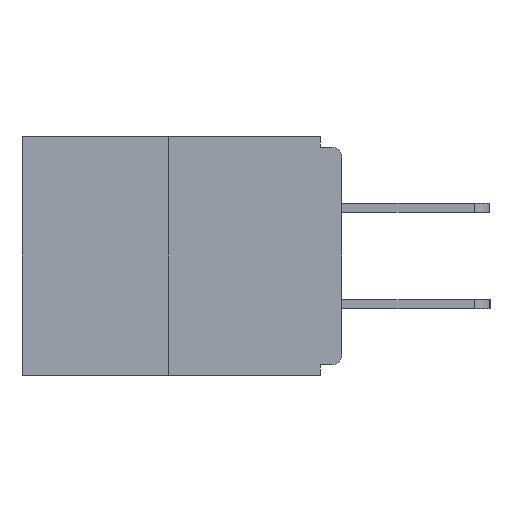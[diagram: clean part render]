
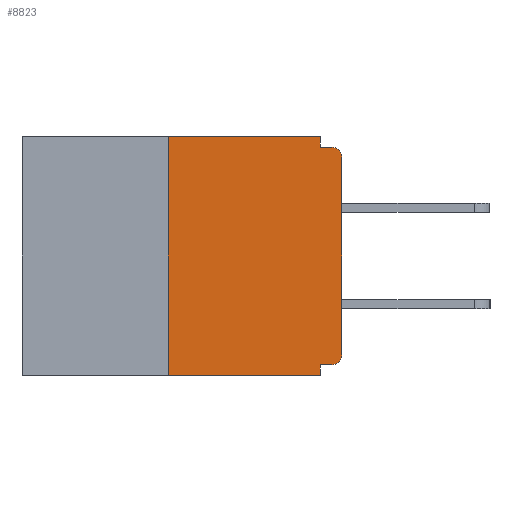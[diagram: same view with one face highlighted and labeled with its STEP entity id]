
A CAD part, left-side view. The second image highlights one B-rep face of the part: STEP entity #8823.
In plain terms, the highlighted planar face has unit normal (-1, 0, 0).
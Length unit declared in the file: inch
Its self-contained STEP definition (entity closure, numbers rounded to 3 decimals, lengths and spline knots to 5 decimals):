
#463 = ORIENTED_EDGE ( 'NONE', *, *, #13800, .T. ) ;
#573 = CARTESIAN_POINT ( 'NONE',  ( 0., 0.46, -0.343 ) ) ;
#720 = ORIENTED_EDGE ( 'NONE', *, *, #5041, .F. ) ;
#728 = ORIENTED_EDGE ( 'NONE', *, *, #3603, .F. ) ;
#1211 = EDGE_CURVE ( 'NONE', #15769, #4730, #8385, .T. ) ;
#1358 = VECTOR ( 'NONE', #7651, 39.37008 ) ;
#1400 = EDGE_CURVE ( 'NONE', #16374, #4620, #12694, .T. ) ;
#1928 = AXIS2_PLACEMENT_3D ( 'NONE', #2084, #3474, #12201 ) ;
#1945 = CARTESIAN_POINT ( 'NONE',  ( 0., 0.031, 0. ) ) ;
#1962 = CARTESIAN_POINT ( 'NONE',  ( 0., 0.46, 0. ) ) ;
#2084 = CARTESIAN_POINT ( 'NONE',  ( 0., 0.015, -0.03 ) ) ;
#2176 = CARTESIAN_POINT ( 'NONE',  ( 0., 0.015, -0.015 ) ) ;
#2355 = CARTESIAN_POINT ( 'NONE',  ( 0., 0., 0. ) ) ;
#3474 = DIRECTION ( 'NONE',  ( -1., 0., 0. ) ) ;
#3556 = ORIENTED_EDGE ( 'NONE', *, *, #1211, .F. ) ;
#3603 = EDGE_CURVE ( 'NONE', #3854, #11603, #16683, .T. ) ;
#3669 = AXIS2_PLACEMENT_3D ( 'NONE', #1962, #14947, #13586 ) ;
#3854 = VERTEX_POINT ( 'NONE', #12225 ) ;
#3891 = VECTOR ( 'NONE', #6583, 39.37008 ) ;
#3928 = ORIENTED_EDGE ( 'NONE', *, *, #1400, .F. ) ;
#3989 = VECTOR ( 'NONE', #10541, 39.37008 ) ;
#4189 = EDGE_CURVE ( 'NONE', #9098, #9670, #17093, .T. ) ;
#4620 = VERTEX_POINT ( 'NONE', #7438 ) ;
#4653 = DIRECTION ( 'NONE',  ( 0., -1., 0. ) ) ;
#4730 = VERTEX_POINT ( 'NONE', #2176 ) ;
#5007 = ORIENTED_EDGE ( 'NONE', *, *, #9114, .F. ) ;
#5041 = EDGE_CURVE ( 'NONE', #4620, #15769, #7080, .T. ) ;
#5430 = VECTOR ( 'NONE', #4653, 39.37008 ) ;
#5467 = CARTESIAN_POINT ( 'NONE',  ( 0., 0.031, -0.015 ) ) ;
#6130 = CARTESIAN_POINT ( 'NONE',  ( 0., 0.46, 0. ) ) ;
#6378 = CIRCLE ( 'NONE', #1928, 0.015 ) ;
#6583 = DIRECTION ( 'NONE',  ( 0., 0., 1. ) ) ;
#6931 = CARTESIAN_POINT ( 'NONE',  ( 0., 0., -0.03 ) ) ;
#6981 = CARTESIAN_POINT ( 'NONE',  ( 0., 0.015, -0.313 ) ) ;
#7080 = LINE ( 'NONE', #1945, #3989 ) ;
#7129 = DIRECTION ( 'NONE',  ( 0., 0., 1. ) ) ;
#7212 = DIRECTION ( 'NONE',  ( 0., -1., 0. ) ) ;
#7337 = CARTESIAN_POINT ( 'NONE',  ( 0., 0.25, 0. ) ) ;
#7438 = CARTESIAN_POINT ( 'NONE',  ( 0., 0.031, 0. ) ) ;
#7651 = DIRECTION ( 'NONE',  ( 0., 0., -1. ) ) ;
#8385 = LINE ( 'NONE', #8486, #15636 ) ;
#8486 = CARTESIAN_POINT ( 'NONE',  ( 0., 0., -0.015 ) ) ;
#8823 = ADVANCED_FACE ( 'NONE', ( #13181 ), #9329, .F. ) ;
#9022 = ORIENTED_EDGE ( 'NONE', *, *, #15590, .T. ) ;
#9098 = VERTEX_POINT ( 'NONE', #9896 ) ;
#9114 = EDGE_CURVE ( 'NONE', #9098, #3854, #13157, .T. ) ;
#9329 = PLANE ( 'NONE',  #3669 ) ;
#9557 = CARTESIAN_POINT ( 'NONE',  ( 0., 0.031, -0.343 ) ) ;
#9670 = VERTEX_POINT ( 'NONE', #9859 ) ;
#9690 = ORIENTED_EDGE ( 'NONE', *, *, #18052, .F. ) ;
#9859 = CARTESIAN_POINT ( 'NONE',  ( 0., 0., -0.313 ) ) ;
#9896 = CARTESIAN_POINT ( 'NONE',  ( 0., 0.015, -0.328 ) ) ;
#9960 = DIRECTION ( 'NONE',  ( 0., 1., 0. ) ) ;
#10215 = LINE ( 'NONE', #2355, #3891 ) ;
#10449 = DIRECTION ( 'NONE',  ( 0., -1., 0. ) ) ;
#10541 = DIRECTION ( 'NONE',  ( 0., 0., -1. ) ) ;
#11110 = CARTESIAN_POINT ( 'NONE',  ( 0., 0.25, -0.343 ) ) ;
#11234 = LINE ( 'NONE', #7337, #13263 ) ;
#11603 = VERTEX_POINT ( 'NONE', #9557 ) ;
#12201 = DIRECTION ( 'NONE',  ( 0., 0., -1. ) ) ;
#12225 = CARTESIAN_POINT ( 'NONE',  ( 0., 0.031, -0.328 ) ) ;
#12694 = LINE ( 'NONE', #6130, #5430 ) ;
#12856 = DIRECTION ( 'NONE',  ( 0., 0., -1. ) ) ;
#13157 = LINE ( 'NONE', #15706, #13609 ) ;
#13181 = FACE_OUTER_BOUND ( 'NONE', #14236, .T. ) ;
#13211 = VERTEX_POINT ( 'NONE', #11110 ) ;
#13248 = VERTEX_POINT ( 'NONE', #6931 ) ;
#13263 = VECTOR ( 'NONE', #7129, 39.37008 ) ;
#13519 = VECTOR ( 'NONE', #10449, 39.37008 ) ;
#13586 = DIRECTION ( 'NONE',  ( 0., 0., -1. ) ) ;
#13609 = VECTOR ( 'NONE', #9960, 39.37008 ) ;
#13800 = EDGE_CURVE ( 'NONE', #13248, #4730, #6378, .T. ) ;
#14100 = DIRECTION ( 'NONE',  ( -1., 0., 0. ) ) ;
#14236 = EDGE_LOOP ( 'NONE', ( #3928, #9690, #15459, #728, #5007, #16792, #9022, #463, #3556, #720 ) ) ;
#14947 = DIRECTION ( 'NONE',  ( 1., 0., 0. ) ) ;
#15305 = LINE ( 'NONE', #573, #13519 ) ;
#15459 = ORIENTED_EDGE ( 'NONE', *, *, #17353, .T. ) ;
#15515 = AXIS2_PLACEMENT_3D ( 'NONE', #6981, #14100, #12856 ) ;
#15590 = EDGE_CURVE ( 'NONE', #9670, #13248, #10215, .T. ) ;
#15636 = VECTOR ( 'NONE', #7212, 39.37008 ) ;
#15706 = CARTESIAN_POINT ( 'NONE',  ( 0., 0., -0.328 ) ) ;
#15740 = CARTESIAN_POINT ( 'NONE',  ( 0., 0.25, 0. ) ) ;
#15769 = VERTEX_POINT ( 'NONE', #5467 ) ;
#16374 = VERTEX_POINT ( 'NONE', #15740 ) ;
#16683 = LINE ( 'NONE', #17595, #1358 ) ;
#16792 = ORIENTED_EDGE ( 'NONE', *, *, #4189, .T. ) ;
#17093 = CIRCLE ( 'NONE', #15515, 0.015 ) ;
#17353 = EDGE_CURVE ( 'NONE', #13211, #11603, #15305, .T. ) ;
#17595 = CARTESIAN_POINT ( 'NONE',  ( 0., 0.031, -0.343 ) ) ;
#18052 = EDGE_CURVE ( 'NONE', #13211, #16374, #11234, .T. ) ;
